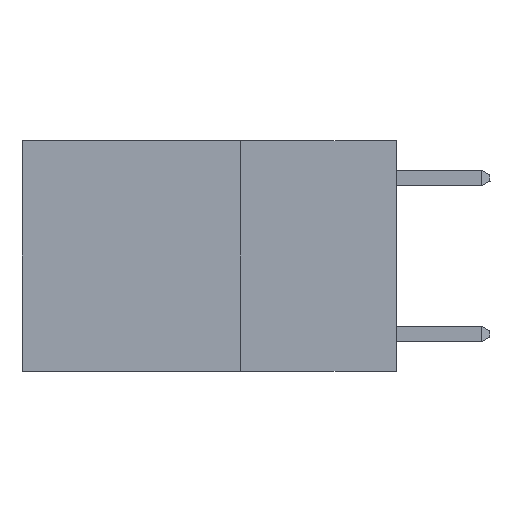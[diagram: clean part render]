
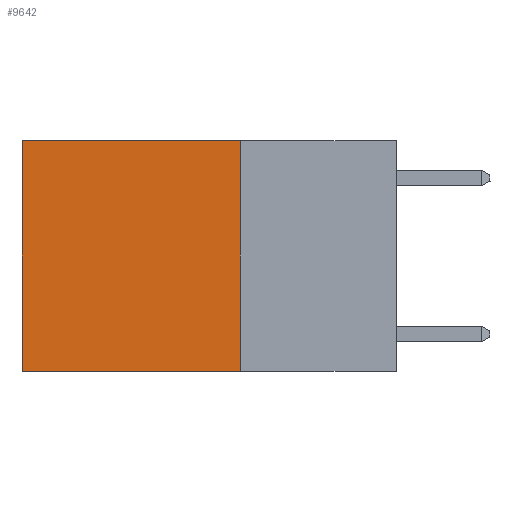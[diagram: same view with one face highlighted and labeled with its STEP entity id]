
A CAD part, left-side view. The second image highlights one B-rep face of the part: STEP entity #9642.
In plain terms, the highlighted planar face has unit normal (-1, 0, 0).
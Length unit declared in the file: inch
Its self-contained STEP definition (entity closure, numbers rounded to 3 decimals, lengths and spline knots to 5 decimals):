
#227 = CARTESIAN_POINT ( 'NONE',  ( 0.2625, 0.6, 0. ) ) ;
#322 = ORIENTED_EDGE ( 'NONE', *, *, #6557, .F. ) ;
#646 = CARTESIAN_POINT ( 'NONE',  ( 0.2625, 0.25, 0. ) ) ;
#704 = VERTEX_POINT ( 'NONE', #3542 ) ;
#919 = LINE ( 'NONE', #1105, #6778 ) ;
#1105 = CARTESIAN_POINT ( 'NONE',  ( 0.2625, 0.25, -0.37 ) ) ;
#1178 = EDGE_CURVE ( 'NONE', #9800, #6865, #8629, .T. ) ;
#1413 = VECTOR ( 'NONE', #7595, 39.37008 ) ;
#1464 = PLANE ( 'NONE',  #3729 ) ;
#1507 = EDGE_CURVE ( 'NONE', #704, #8903, #919, .T. ) ;
#1593 = CARTESIAN_POINT ( 'NONE',  ( 0.2625, 0.6, -0.37 ) ) ;
#1915 = DIRECTION ( 'NONE',  ( 0., 0., -1. ) ) ;
#2269 = CARTESIAN_POINT ( 'NONE',  ( 0.2625, 0.25, 0. ) ) ;
#2304 = DIRECTION ( 'NONE',  ( 1., 0., 0. ) ) ;
#2328 = EDGE_CURVE ( 'NONE', #6865, #8903, #4732, .T. ) ;
#2335 = CARTESIAN_POINT ( 'NONE',  ( 0.2625, 0.6, 0. ) ) ;
#3542 = CARTESIAN_POINT ( 'NONE',  ( 0.2625, 0.25, -0.37 ) ) ;
#3729 = AXIS2_PLACEMENT_3D ( 'NONE', #2269, #2304, #1915 ) ;
#3802 = CARTESIAN_POINT ( 'NONE',  ( 0.2625, 0.25, 0. ) ) ;
#4171 = DIRECTION ( 'NONE',  ( 0., 1., 0. ) ) ;
#4523 = VECTOR ( 'NONE', #6847, 39.37008 ) ;
#4732 = LINE ( 'NONE', #2335, #6501 ) ;
#5101 = ORIENTED_EDGE ( 'NONE', *, *, #1178, .T. ) ;
#5381 = ORIENTED_EDGE ( 'NONE', *, *, #2328, .T. ) ;
#6332 = FACE_OUTER_BOUND ( 'NONE', #6838, .T. ) ;
#6501 = VECTOR ( 'NONE', #6911, 39.37008 ) ;
#6557 = EDGE_CURVE ( 'NONE', #9800, #704, #9570, .T. ) ;
#6778 = VECTOR ( 'NONE', #4171, 39.37008 ) ;
#6838 = EDGE_LOOP ( 'NONE', ( #5381, #7757, #322, #5101 ) ) ;
#6847 = DIRECTION ( 'NONE',  ( 0., 1., 0. ) ) ;
#6865 = VERTEX_POINT ( 'NONE', #227 ) ;
#6911 = DIRECTION ( 'NONE',  ( 0., 0., -1. ) ) ;
#7595 = DIRECTION ( 'NONE',  ( 0., 0., -1. ) ) ;
#7603 = CARTESIAN_POINT ( 'NONE',  ( 0.2625, 0.25, 0. ) ) ;
#7757 = ORIENTED_EDGE ( 'NONE', *, *, #1507, .F. ) ;
#8629 = LINE ( 'NONE', #646, #4523 ) ;
#8903 = VERTEX_POINT ( 'NONE', #1593 ) ;
#9570 = LINE ( 'NONE', #3802, #1413 ) ;
#9642 = ADVANCED_FACE ( 'NONE', ( #6332 ), #1464, .F. ) ;
#9800 = VERTEX_POINT ( 'NONE', #7603 ) ;
